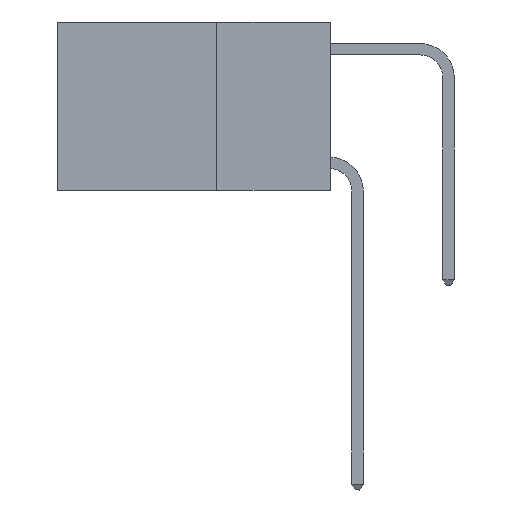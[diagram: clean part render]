
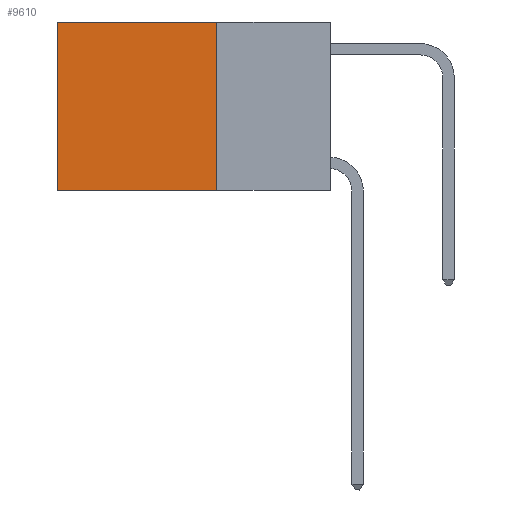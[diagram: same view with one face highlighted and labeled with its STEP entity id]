
A CAD part, left-side view. The second image highlights one B-rep face of the part: STEP entity #9610.
In plain terms, the highlighted planar face has unit normal (-1, 0, 0).
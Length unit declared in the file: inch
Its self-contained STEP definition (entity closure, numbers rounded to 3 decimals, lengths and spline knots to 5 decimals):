
#110 = ORIENTED_EDGE ( 'NONE', *, *, #1720, .T. ) ;
#248 = VECTOR ( 'NONE', #3408, 39.37008 ) ;
#456 = VERTEX_POINT ( 'NONE', #3084 ) ;
#1584 = DIRECTION ( 'NONE',  ( 0., 1., 0. ) ) ;
#1720 = EDGE_CURVE ( 'NONE', #6159, #6104, #4078, .T. ) ;
#2130 = AXIS2_PLACEMENT_3D ( 'NONE', #3697, #20020, #15050 ) ;
#3084 = CARTESIAN_POINT ( 'NONE',  ( 0.2625, 0.25, -0.37 ) ) ;
#3408 = DIRECTION ( 'NONE',  ( 0., 1., 0. ) ) ;
#3697 = CARTESIAN_POINT ( 'NONE',  ( 0.2625, 0.25, 0. ) ) ;
#4078 = LINE ( 'NONE', #12924, #20249 ) ;
#4326 = CARTESIAN_POINT ( 'NONE',  ( 0.2625, 0.6, 0. ) ) ;
#4452 = ORIENTED_EDGE ( 'NONE', *, *, #18151, .F. ) ;
#5023 = VECTOR ( 'NONE', #18233, 39.37008 ) ;
#5127 = VECTOR ( 'NONE', #1584, 39.37008 ) ;
#5183 = EDGE_CURVE ( 'NONE', #13288, #6159, #9929, .T. ) ;
#6104 = VERTEX_POINT ( 'NONE', #10509 ) ;
#6159 = VERTEX_POINT ( 'NONE', #4326 ) ;
#6287 = CARTESIAN_POINT ( 'NONE',  ( 0.2625, 0.25, 0. ) ) ;
#6547 = CARTESIAN_POINT ( 'NONE',  ( 0.2625, 0.25, -0.37 ) ) ;
#7173 = ORIENTED_EDGE ( 'NONE', *, *, #9447, .F. ) ;
#8602 = LINE ( 'NONE', #12993, #5023 ) ;
#9447 = EDGE_CURVE ( 'NONE', #456, #6104, #12636, .T. ) ;
#9610 = ADVANCED_FACE ( 'NONE', ( #20479 ), #16549, .F. ) ;
#9929 = LINE ( 'NONE', #14565, #5127 ) ;
#10509 = CARTESIAN_POINT ( 'NONE',  ( 0.2625, 0.6, -0.37 ) ) ;
#12636 = LINE ( 'NONE', #6547, #248 ) ;
#12924 = CARTESIAN_POINT ( 'NONE',  ( 0.2625, 0.6, 0. ) ) ;
#12993 = CARTESIAN_POINT ( 'NONE',  ( 0.2625, 0.25, 0. ) ) ;
#13288 = VERTEX_POINT ( 'NONE', #6287 ) ;
#14565 = CARTESIAN_POINT ( 'NONE',  ( 0.2625, 0.25, 0. ) ) ;
#15050 = DIRECTION ( 'NONE',  ( 0., 0., -1. ) ) ;
#16549 = PLANE ( 'NONE',  #2130 ) ;
#17527 = EDGE_LOOP ( 'NONE', ( #110, #7173, #4452, #19713 ) ) ;
#18151 = EDGE_CURVE ( 'NONE', #13288, #456, #8602, .T. ) ;
#18233 = DIRECTION ( 'NONE',  ( 0., 0., -1. ) ) ;
#19713 = ORIENTED_EDGE ( 'NONE', *, *, #5183, .T. ) ;
#19896 = DIRECTION ( 'NONE',  ( 0., 0., -1. ) ) ;
#20020 = DIRECTION ( 'NONE',  ( 1., 0., 0. ) ) ;
#20249 = VECTOR ( 'NONE', #19896, 39.37008 ) ;
#20479 = FACE_OUTER_BOUND ( 'NONE', #17527, .T. ) ;
